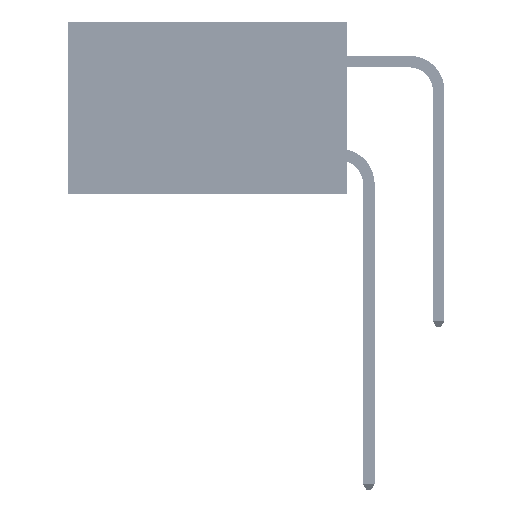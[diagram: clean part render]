
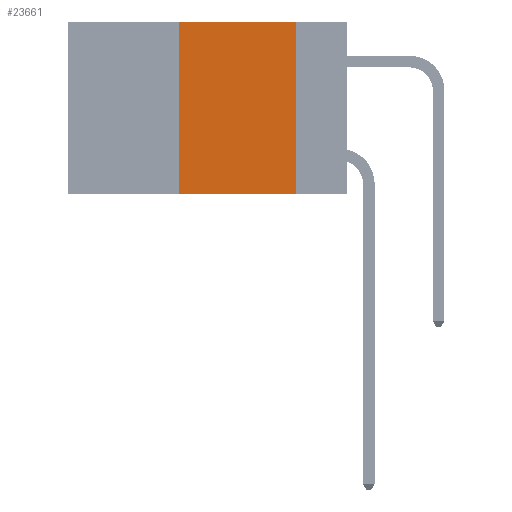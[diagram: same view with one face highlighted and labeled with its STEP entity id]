
A CAD part, left-side view. The second image highlights one B-rep face of the part: STEP entity #23661.
In plain terms, the highlighted planar face has unit normal (-1, 0, 0).
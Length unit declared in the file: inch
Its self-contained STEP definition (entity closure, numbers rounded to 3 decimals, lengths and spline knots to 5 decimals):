
#1336 = LINE ( 'NONE', #32351, #30421 ) ;
#2811 = CARTESIAN_POINT ( 'NONE',  ( 0., 0.11, 0. ) ) ;
#2816 = CARTESIAN_POINT ( 'NONE',  ( 0., 0.6, -0.37 ) ) ;
#7287 = CARTESIAN_POINT ( 'NONE',  ( 0., 0.36, 0. ) ) ;
#7424 = VERTEX_POINT ( 'NONE', #46285 ) ;
#10571 = DIRECTION ( 'NONE',  ( 0., -1., 0. ) ) ;
#11718 = EDGE_CURVE ( 'NONE', #12842, #24062, #35498, .T. ) ;
#12842 = VERTEX_POINT ( 'NONE', #34398 ) ;
#14106 = AXIS2_PLACEMENT_3D ( 'NONE', #18086, #43437, #21689 ) ;
#15689 = EDGE_CURVE ( 'NONE', #24304, #24062, #43664, .T. ) ;
#15804 = ORIENTED_EDGE ( 'NONE', *, *, #25641, .F. ) ;
#18086 = CARTESIAN_POINT ( 'NONE',  ( 0., 0.6, 0. ) ) ;
#18286 = ORIENTED_EDGE ( 'NONE', *, *, #15689, .F. ) ;
#20982 = DIRECTION ( 'NONE',  ( 0., -1., 0. ) ) ;
#21689 = DIRECTION ( 'NONE',  ( 0., 0., -1. ) ) ;
#23661 = ADVANCED_FACE ( 'NONE', ( #46440 ), #28863, .F. ) ;
#24062 = VERTEX_POINT ( 'NONE', #27020 ) ;
#24188 = CARTESIAN_POINT ( 'NONE',  ( 0., 0.11, 0. ) ) ;
#24304 = VERTEX_POINT ( 'NONE', #2811 ) ;
#25641 = EDGE_CURVE ( 'NONE', #7424, #24304, #1336, .T. ) ;
#27020 = CARTESIAN_POINT ( 'NONE',  ( 0., 0.11, -0.37 ) ) ;
#28863 = PLANE ( 'NONE',  #14106 ) ;
#29279 = EDGE_LOOP ( 'NONE', ( #18286, #15804, #41329, #30561 ) ) ;
#30421 = VECTOR ( 'NONE', #10571, 39.37008 ) ;
#30561 = ORIENTED_EDGE ( 'NONE', *, *, #11718, .T. ) ;
#32194 = VECTOR ( 'NONE', #36380, 39.37008 ) ;
#32351 = CARTESIAN_POINT ( 'NONE',  ( 0., 0.6, 0. ) ) ;
#34398 = CARTESIAN_POINT ( 'NONE',  ( 0., 0.36, -0.37 ) ) ;
#35498 = LINE ( 'NONE', #2816, #43954 ) ;
#36380 = DIRECTION ( 'NONE',  ( 0., 0., 1. ) ) ;
#40249 = VECTOR ( 'NONE', #42275, 39.37008 ) ;
#41329 = ORIENTED_EDGE ( 'NONE', *, *, #43358, .F. ) ;
#41785 = LINE ( 'NONE', #7287, #32194 ) ;
#42275 = DIRECTION ( 'NONE',  ( 0., 0., -1. ) ) ;
#43358 = EDGE_CURVE ( 'NONE', #12842, #7424, #41785, .T. ) ;
#43437 = DIRECTION ( 'NONE',  ( 1., 0., 0. ) ) ;
#43664 = LINE ( 'NONE', #24188, #40249 ) ;
#43954 = VECTOR ( 'NONE', #20982, 39.37008 ) ;
#46285 = CARTESIAN_POINT ( 'NONE',  ( 0., 0.36, 0. ) ) ;
#46440 = FACE_OUTER_BOUND ( 'NONE', #29279, .T. ) ;
